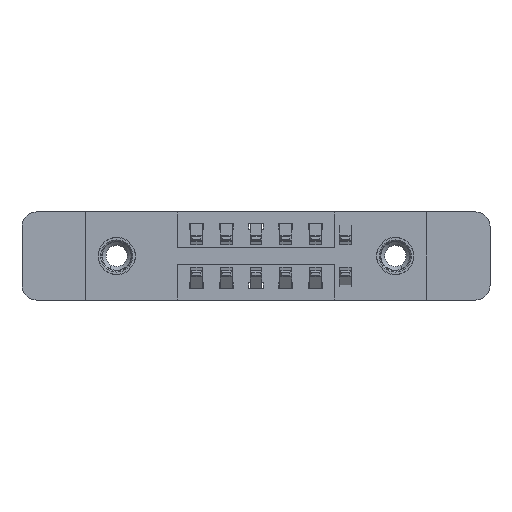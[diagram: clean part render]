
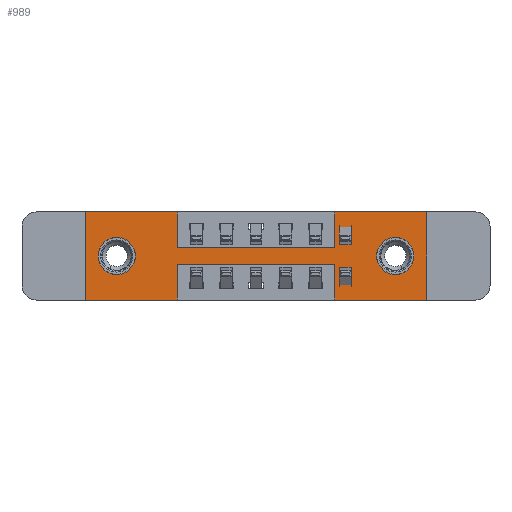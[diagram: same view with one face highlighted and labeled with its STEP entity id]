
A CAD part, front view. The second image highlights one B-rep face of the part: STEP entity #989.
In plain terms, the highlighted planar face has unit normal (0, -1, 0).
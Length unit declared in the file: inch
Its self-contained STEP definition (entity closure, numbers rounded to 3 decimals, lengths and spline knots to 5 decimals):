
#118 = DIRECTION ( 'NONE',  ( 0., 1., 0. ) ) ;
#247 = LINE ( 'NONE', #1243, #12067 ) ;
#460 = VERTEX_POINT ( 'NONE', #8002 ) ;
#463 = LINE ( 'NONE', #4865, #6053 ) ;
#468 = CARTESIAN_POINT ( 'NONE',  ( 0.3875, 0., -0.37 ) ) ;
#508 = ORIENTED_EDGE ( 'NONE', *, *, #7959, .T. ) ;
#716 = DIRECTION ( 'NONE',  ( 0., 1., 0. ) ) ;
#806 = FACE_BOUND ( 'NONE', #12705, .T. ) ;
#878 = FACE_OUTER_BOUND ( 'NONE', #9754, .T. ) ;
#989 = ADVANCED_FACE ( 'NONE', ( #806, #2859, #878 ), #5204, .T. ) ;
#1076 = AXIS2_PLACEMENT_3D ( 'NONE', #8236, #716, #1635 ) ;
#1243 = CARTESIAN_POINT ( 'NONE',  ( 0., 0., -0.37 ) ) ;
#1311 = ORIENTED_EDGE ( 'NONE', *, *, #11048, .F. ) ;
#1586 = DIRECTION ( 'NONE',  ( 0., 1., 0. ) ) ;
#1635 = DIRECTION ( 'NONE',  ( 0., 0., 1. ) ) ;
#1657 = AXIS2_PLACEMENT_3D ( 'NONE', #11631, #6070, #7123 ) ;
#1761 = EDGE_CURVE ( 'NONE', #9166, #8997, #4786, .T. ) ;
#2221 = DIRECTION ( 'NONE',  ( -1., 0., 0. ) ) ;
#2504 = EDGE_CURVE ( 'NONE', #7857, #7617, #463, .T. ) ;
#2565 = ORIENTED_EDGE ( 'NONE', *, *, #11345, .T. ) ;
#2626 = VECTOR ( 'NONE', #11087, 39.37008 ) ;
#2750 = CIRCLE ( 'NONE', #9549, 0.078 ) ;
#2834 = CARTESIAN_POINT ( 'NONE',  ( 0.3875, 0., -0.22 ) ) ;
#2859 = FACE_BOUND ( 'NONE', #8688, .T. ) ;
#2926 = ORIENTED_EDGE ( 'NONE', *, *, #5093, .T. ) ;
#2927 = VECTOR ( 'NONE', #3445, 39.37008 ) ;
#3002 = ORIENTED_EDGE ( 'NONE', *, *, #10085, .T. ) ;
#3165 = DIRECTION ( 'NONE',  ( 0., 0., 1. ) ) ;
#3445 = DIRECTION ( 'NONE',  ( 0., 0., -1. ) ) ;
#3458 = DIRECTION ( 'NONE',  ( 0., 0., -1. ) ) ;
#3629 = VERTEX_POINT ( 'NONE', #6081 ) ;
#3660 = DIRECTION ( 'NONE',  ( 1., 0., 0. ) ) ;
#3689 = CIRCLE ( 'NONE', #4831, 0.078 ) ;
#3698 = EDGE_CURVE ( 'NONE', #460, #8109, #10802, .T. ) ;
#3789 = ORIENTED_EDGE ( 'NONE', *, *, #13860, .F. ) ;
#4146 = CARTESIAN_POINT ( 'NONE',  ( 0., 0., -0.37 ) ) ;
#4160 = CARTESIAN_POINT ( 'NONE',  ( 0.3875, 0., 0. ) ) ;
#4337 = LINE ( 'NONE', #12962, #6746 ) ;
#4494 = EDGE_CURVE ( 'NONE', #5128, #460, #8056, .T. ) ;
#4569 = VERTEX_POINT ( 'NONE', #468 ) ;
#4651 = CARTESIAN_POINT ( 'NONE',  ( 1.0475, 0., 0. ) ) ;
#4786 = LINE ( 'NONE', #4651, #2626 ) ;
#4831 = AXIS2_PLACEMENT_3D ( 'NONE', #11937, #118, #12878 ) ;
#4865 = CARTESIAN_POINT ( 'NONE',  ( 0.3875, 0., 0. ) ) ;
#5010 = LINE ( 'NONE', #11509, #8744 ) ;
#5052 = ORIENTED_EDGE ( 'NONE', *, *, #3698, .F. ) ;
#5093 = EDGE_CURVE ( 'NONE', #6155, #3629, #2750, .T. ) ;
#5128 = VERTEX_POINT ( 'NONE', #12635 ) ;
#5204 = PLANE ( 'NONE',  #6954 ) ;
#5230 = LINE ( 'NONE', #10674, #7093 ) ;
#5281 = CARTESIAN_POINT ( 'NONE',  ( 1.3025, 0., -0.263 ) ) ;
#5348 = CARTESIAN_POINT ( 'NONE',  ( 0., 0., 0. ) ) ;
#5383 = DIRECTION ( 'NONE',  ( -1., 0., 0. ) ) ;
#5538 = CIRCLE ( 'NONE', #1657, 0.078 ) ;
#6053 = VECTOR ( 'NONE', #11292, 39.37008 ) ;
#6070 = DIRECTION ( 'NONE',  ( 0., 1., 0. ) ) ;
#6081 = CARTESIAN_POINT ( 'NONE',  ( 0.1325, 0., -0.263 ) ) ;
#6155 = VERTEX_POINT ( 'NONE', #7163 ) ;
#6478 = CARTESIAN_POINT ( 'NONE',  ( 1.3025, 0., -0.107 ) ) ;
#6515 = CARTESIAN_POINT ( 'NONE',  ( 1.0475, 0., -0.22 ) ) ;
#6715 = ORIENTED_EDGE ( 'NONE', *, *, #9868, .F. ) ;
#6726 = CARTESIAN_POINT ( 'NONE',  ( 1.0475, 0., 0. ) ) ;
#6746 = VECTOR ( 'NONE', #3458, 39.37008 ) ;
#6855 = LINE ( 'NONE', #11235, #12104 ) ;
#6954 = AXIS2_PLACEMENT_3D ( 'NONE', #8402, #13635, #13847 ) ;
#7022 = VERTEX_POINT ( 'NONE', #12555 ) ;
#7093 = VECTOR ( 'NONE', #3165, 39.37008 ) ;
#7123 = DIRECTION ( 'NONE',  ( 0., 0., -1. ) ) ;
#7163 = CARTESIAN_POINT ( 'NONE',  ( 0.1325, 0., -0.107 ) ) ;
#7271 = DIRECTION ( 'NONE',  ( -1., 0., 0. ) ) ;
#7454 = ORIENTED_EDGE ( 'NONE', *, *, #9872, .F. ) ;
#7617 = VERTEX_POINT ( 'NONE', #8584 ) ;
#7857 = VERTEX_POINT ( 'NONE', #4160 ) ;
#7921 = ORIENTED_EDGE ( 'NONE', *, *, #13761, .F. ) ;
#7959 = EDGE_CURVE ( 'NONE', #11568, #11527, #3689, .T. ) ;
#8002 = CARTESIAN_POINT ( 'NONE',  ( 1.435, 0., -0.37 ) ) ;
#8056 = LINE ( 'NONE', #9978, #2927 ) ;
#8109 = VERTEX_POINT ( 'NONE', #9971 ) ;
#8156 = VERTEX_POINT ( 'NONE', #9105 ) ;
#8236 = CARTESIAN_POINT ( 'NONE',  ( 0.1325, 0., -0.185 ) ) ;
#8355 = CARTESIAN_POINT ( 'NONE',  ( 0., 0., 0. ) ) ;
#8402 = CARTESIAN_POINT ( 'NONE',  ( 0., 0., -0.37 ) ) ;
#8514 = VERTEX_POINT ( 'NONE', #2834 ) ;
#8584 = CARTESIAN_POINT ( 'NONE',  ( 0.3875, 0., -0.15 ) ) ;
#8688 = EDGE_LOOP ( 'NONE', ( #2926, #3002 ) ) ;
#8744 = VECTOR ( 'NONE', #12584, 39.37008 ) ;
#8850 = EDGE_CURVE ( 'NONE', #8514, #4569, #4337, .T. ) ;
#8997 = VERTEX_POINT ( 'NONE', #6726 ) ;
#9105 = CARTESIAN_POINT ( 'NONE',  ( 0., 0., 0. ) ) ;
#9166 = VERTEX_POINT ( 'NONE', #11372 ) ;
#9401 = LINE ( 'NONE', #10464, #10053 ) ;
#9540 = VERTEX_POINT ( 'NONE', #6515 ) ;
#9549 = AXIS2_PLACEMENT_3D ( 'NONE', #10515, #1586, #13570 ) ;
#9579 = DIRECTION ( 'NONE',  ( 1., 0., 0. ) ) ;
#9616 = DIRECTION ( 'NONE',  ( 1., 0., 0. ) ) ;
#9754 = EDGE_LOOP ( 'NONE', ( #10164, #7454, #1311, #5052, #13947, #13903, #10661, #7921, #13568, #3789, #6715, #13524 ) ) ;
#9868 = EDGE_CURVE ( 'NONE', #7022, #8156, #5010, .T. ) ;
#9872 = EDGE_CURVE ( 'NONE', #9540, #8514, #9401, .T. ) ;
#9971 = CARTESIAN_POINT ( 'NONE',  ( 1.0475, 0., -0.37 ) ) ;
#9978 = CARTESIAN_POINT ( 'NONE',  ( 1.435, 0., 0. ) ) ;
#10053 = VECTOR ( 'NONE', #7271, 39.37008 ) ;
#10085 = EDGE_CURVE ( 'NONE', #3629, #6155, #10554, .T. ) ;
#10164 = ORIENTED_EDGE ( 'NONE', *, *, #8850, .F. ) ;
#10464 = CARTESIAN_POINT ( 'NONE',  ( 0.3875, 0., -0.22 ) ) ;
#10515 = CARTESIAN_POINT ( 'NONE',  ( 0.1325, 0., -0.185 ) ) ;
#10554 = CIRCLE ( 'NONE', #1076, 0.078 ) ;
#10661 = ORIENTED_EDGE ( 'NONE', *, *, #1761, .F. ) ;
#10674 = CARTESIAN_POINT ( 'NONE',  ( 1.0475, 0., -0.37 ) ) ;
#10754 = VECTOR ( 'NONE', #9579, 39.37008 ) ;
#10802 = LINE ( 'NONE', #4146, #11485 ) ;
#10851 = LINE ( 'NONE', #5348, #10754 ) ;
#11048 = EDGE_CURVE ( 'NONE', #8109, #9540, #5230, .T. ) ;
#11087 = DIRECTION ( 'NONE',  ( 0., 0., 1. ) ) ;
#11235 = CARTESIAN_POINT ( 'NONE',  ( 0.3875, 0., -0.15 ) ) ;
#11292 = DIRECTION ( 'NONE',  ( 0., 0., -1. ) ) ;
#11345 = EDGE_CURVE ( 'NONE', #11527, #11568, #5538, .T. ) ;
#11372 = CARTESIAN_POINT ( 'NONE',  ( 1.0475, 0., -0.15 ) ) ;
#11485 = VECTOR ( 'NONE', #2221, 39.37008 ) ;
#11509 = CARTESIAN_POINT ( 'NONE',  ( 0., 0., 0. ) ) ;
#11527 = VERTEX_POINT ( 'NONE', #6478 ) ;
#11568 = VERTEX_POINT ( 'NONE', #5281 ) ;
#11584 = LINE ( 'NONE', #8355, #13033 ) ;
#11631 = CARTESIAN_POINT ( 'NONE',  ( 1.3025, 0., -0.185 ) ) ;
#11937 = CARTESIAN_POINT ( 'NONE',  ( 1.3025, 0., -0.185 ) ) ;
#12067 = VECTOR ( 'NONE', #5383, 39.37008 ) ;
#12104 = VECTOR ( 'NONE', #3660, 39.37008 ) ;
#12282 = EDGE_CURVE ( 'NONE', #4569, #7022, #247, .T. ) ;
#12555 = CARTESIAN_POINT ( 'NONE',  ( 0., 0., -0.37 ) ) ;
#12584 = DIRECTION ( 'NONE',  ( 0., 0., 1. ) ) ;
#12635 = CARTESIAN_POINT ( 'NONE',  ( 1.435, 0., 0. ) ) ;
#12705 = EDGE_LOOP ( 'NONE', ( #2565, #508 ) ) ;
#12878 = DIRECTION ( 'NONE',  ( 0., 0., -1. ) ) ;
#12962 = CARTESIAN_POINT ( 'NONE',  ( 0.3875, 0., -0.37 ) ) ;
#13033 = VECTOR ( 'NONE', #9616, 39.37008 ) ;
#13120 = EDGE_CURVE ( 'NONE', #8997, #5128, #10851, .T. ) ;
#13524 = ORIENTED_EDGE ( 'NONE', *, *, #12282, .F. ) ;
#13568 = ORIENTED_EDGE ( 'NONE', *, *, #2504, .F. ) ;
#13570 = DIRECTION ( 'NONE',  ( 0., 0., 1. ) ) ;
#13635 = DIRECTION ( 'NONE',  ( 0., -1., 0. ) ) ;
#13761 = EDGE_CURVE ( 'NONE', #7617, #9166, #6855, .T. ) ;
#13847 = DIRECTION ( 'NONE',  ( 0., 0., -1. ) ) ;
#13860 = EDGE_CURVE ( 'NONE', #8156, #7857, #11584, .T. ) ;
#13903 = ORIENTED_EDGE ( 'NONE', *, *, #13120, .F. ) ;
#13947 = ORIENTED_EDGE ( 'NONE', *, *, #4494, .F. ) ;
